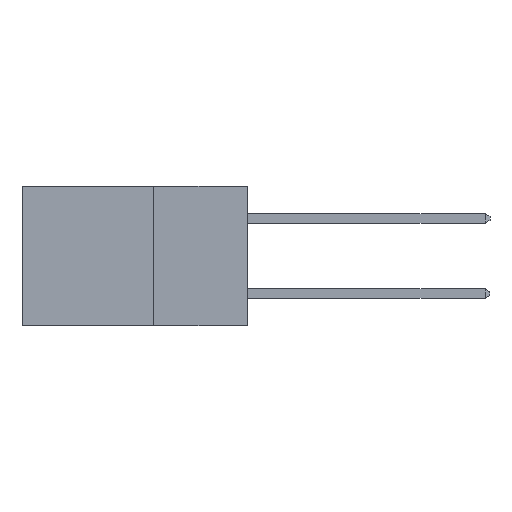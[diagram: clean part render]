
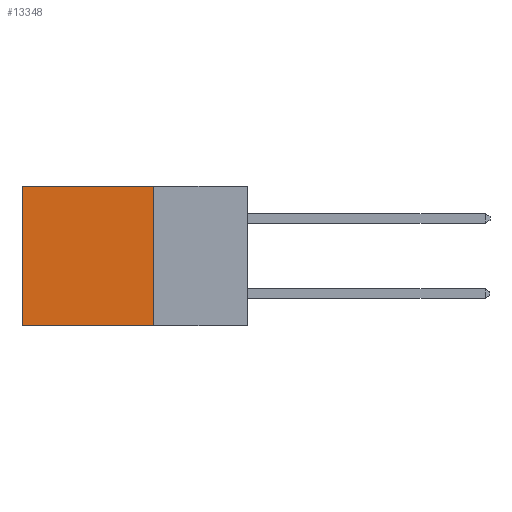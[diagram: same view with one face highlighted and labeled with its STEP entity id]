
A CAD part, left-side view. The second image highlights one B-rep face of the part: STEP entity #13348.
In plain terms, the highlighted planar face has unit normal (-1, 0, 0).
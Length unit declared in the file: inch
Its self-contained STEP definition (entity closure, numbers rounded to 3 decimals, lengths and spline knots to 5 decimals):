
#199 = DIRECTION ( 'NONE',  ( 1., 0., 0. ) ) ;
#266 = LINE ( 'NONE', #14691, #12928 ) ;
#1011 = EDGE_LOOP ( 'NONE', ( #10682, #1997, #6743, #5498 ) ) ;
#1905 = FACE_OUTER_BOUND ( 'NONE', #1011, .T. ) ;
#1911 = DIRECTION ( 'NONE',  ( 0., 0., -1. ) ) ;
#1997 = ORIENTED_EDGE ( 'NONE', *, *, #10125, .F. ) ;
#3115 = CARTESIAN_POINT ( 'NONE',  ( 0.298, 0.6, 0. ) ) ;
#3166 = DIRECTION ( 'NONE',  ( 0., 1., 0. ) ) ;
#3500 = LINE ( 'NONE', #9057, #9397 ) ;
#3812 = CARTESIAN_POINT ( 'NONE',  ( 0.298, 0.6, -0.37 ) ) ;
#4357 = DIRECTION ( 'NONE',  ( 0., 0., -1. ) ) ;
#5288 = CARTESIAN_POINT ( 'NONE',  ( 0.298, 0.6, 0. ) ) ;
#5498 = ORIENTED_EDGE ( 'NONE', *, *, #7630, .T. ) ;
#6559 = AXIS2_PLACEMENT_3D ( 'NONE', #9755, #199, #8653 ) ;
#6743 = ORIENTED_EDGE ( 'NONE', *, *, #11258, .F. ) ;
#7048 = VERTEX_POINT ( 'NONE', #9150 ) ;
#7487 = PLANE ( 'NONE',  #6559 ) ;
#7495 = VERTEX_POINT ( 'NONE', #5288 ) ;
#7629 = LINE ( 'NONE', #13714, #13384 ) ;
#7630 = EDGE_CURVE ( 'NONE', #10216, #7495, #266, .T. ) ;
#8007 = VERTEX_POINT ( 'NONE', #3812 ) ;
#8653 = DIRECTION ( 'NONE',  ( 0., 0., -1. ) ) ;
#9057 = CARTESIAN_POINT ( 'NONE',  ( 0.298, 0.25, 0. ) ) ;
#9150 = CARTESIAN_POINT ( 'NONE',  ( 0.298, 0.25, -0.37 ) ) ;
#9397 = VECTOR ( 'NONE', #1911, 39.37008 ) ;
#9755 = CARTESIAN_POINT ( 'NONE',  ( 0.298, 0.25, 0. ) ) ;
#10061 = EDGE_CURVE ( 'NONE', #7495, #8007, #11734, .T. ) ;
#10125 = EDGE_CURVE ( 'NONE', #7048, #8007, #7629, .T. ) ;
#10216 = VERTEX_POINT ( 'NONE', #12752 ) ;
#10682 = ORIENTED_EDGE ( 'NONE', *, *, #10061, .T. ) ;
#11258 = EDGE_CURVE ( 'NONE', #10216, #7048, #3500, .T. ) ;
#11366 = VECTOR ( 'NONE', #4357, 39.37008 ) ;
#11734 = LINE ( 'NONE', #3115, #11366 ) ;
#12752 = CARTESIAN_POINT ( 'NONE',  ( 0.298, 0.25, 0. ) ) ;
#12928 = VECTOR ( 'NONE', #3166, 39.37008 ) ;
#13348 = ADVANCED_FACE ( 'NONE', ( #1905 ), #7487, .F. ) ;
#13384 = VECTOR ( 'NONE', #14790, 39.37008 ) ;
#13714 = CARTESIAN_POINT ( 'NONE',  ( 0.298, 0.25, -0.37 ) ) ;
#14691 = CARTESIAN_POINT ( 'NONE',  ( 0.298, 0.25, 0. ) ) ;
#14790 = DIRECTION ( 'NONE',  ( 0., 1., 0. ) ) ;
